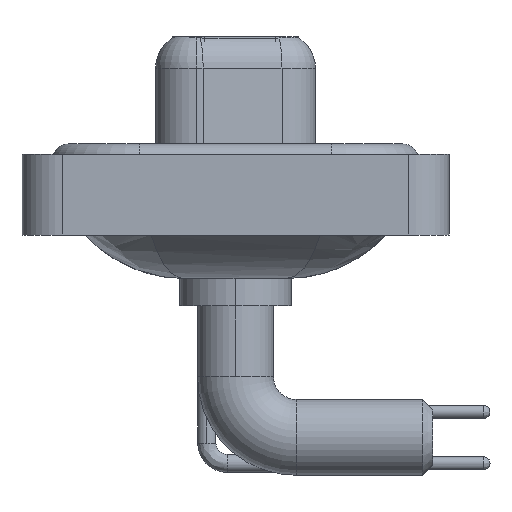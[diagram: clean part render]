
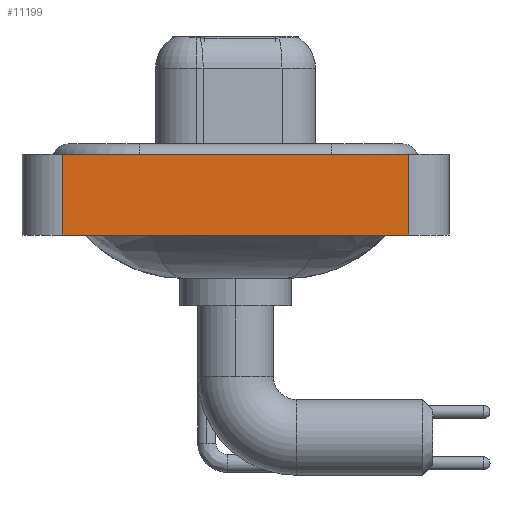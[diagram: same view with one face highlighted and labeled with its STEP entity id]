
A CAD part, left-side view. The second image highlights one B-rep face of the part: STEP entity #11199.
In plain terms, the highlighted planar face has unit normal (-1, 0, 0).
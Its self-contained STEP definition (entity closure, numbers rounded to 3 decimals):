
#631 = VECTOR ( 'NONE', #13515, 1000. ) ;
#1649 = LINE ( 'NONE', #22675, #10372 ) ;
#2010 = DIRECTION ( 'NONE',  ( 0., -1., 0. ) ) ;
#2156 = CARTESIAN_POINT ( 'NONE',  ( -7.35, 8.55, 0.4 ) ) ;
#2305 = VERTEX_POINT ( 'NONE', #13237 ) ;
#2720 = DIRECTION ( 'NONE',  ( 0., 0., 1. ) ) ;
#3395 = EDGE_LOOP ( 'NONE', ( #18081, #11833, #18886, #6422 ) ) ;
#3696 = DIRECTION ( 'NONE',  ( 0., 0., 1. ) ) ;
#4889 = DIRECTION ( 'NONE',  ( 0., -1., 0. ) ) ;
#5348 = LINE ( 'NONE', #7162, #11766 ) ;
#5562 = EDGE_CURVE ( 'NONE', #19245, #2305, #22698, .T. ) ;
#5901 = CARTESIAN_POINT ( 'NONE',  ( -7.35, 8.55, -3.6 ) ) ;
#6056 = CARTESIAN_POINT ( 'NONE',  ( -7.35, -8.55, -3.6 ) ) ;
#6422 = ORIENTED_EDGE ( 'NONE', *, *, #20393, .T. ) ;
#6486 = CARTESIAN_POINT ( 'NONE',  ( -7.35, -8.55, -3.6 ) ) ;
#6576 = CARTESIAN_POINT ( 'NONE',  ( -7.35, -8.55, -3.6 ) ) ;
#6828 = VERTEX_POINT ( 'NONE', #2156 ) ;
#7162 = CARTESIAN_POINT ( 'NONE',  ( -7.35, -8.55, 0.4 ) ) ;
#9732 = CARTESIAN_POINT ( 'NONE',  ( -7.35, -8.55, -3.6 ) ) ;
#10372 = VECTOR ( 'NONE', #3696, 1000. ) ;
#11199 = ADVANCED_FACE ( 'NONE', ( #14770 ), #16617, .T. ) ;
#11508 = VERTEX_POINT ( 'NONE', #5901 ) ;
#11766 = VECTOR ( 'NONE', #2010, 1000. ) ;
#11833 = ORIENTED_EDGE ( 'NONE', *, *, #16425, .F. ) ;
#13062 = DIRECTION ( 'NONE',  ( -1., 0., 0. ) ) ;
#13237 = CARTESIAN_POINT ( 'NONE',  ( -7.35, -8.55, 0.4 ) ) ;
#13515 = DIRECTION ( 'NONE',  ( 0., 0., 1. ) ) ;
#14004 = VECTOR ( 'NONE', #4889, 1000. ) ;
#14770 = FACE_OUTER_BOUND ( 'NONE', #3395, .T. ) ;
#16130 = AXIS2_PLACEMENT_3D ( 'NONE', #6056, #13062, #2720 ) ;
#16425 = EDGE_CURVE ( 'NONE', #6828, #2305, #5348, .T. ) ;
#16617 = PLANE ( 'NONE',  #16130 ) ;
#16948 = LINE ( 'NONE', #9732, #14004 ) ;
#18081 = ORIENTED_EDGE ( 'NONE', *, *, #5562, .T. ) ;
#18108 = EDGE_CURVE ( 'NONE', #11508, #6828, #1649, .T. ) ;
#18886 = ORIENTED_EDGE ( 'NONE', *, *, #18108, .F. ) ;
#19245 = VERTEX_POINT ( 'NONE', #6576 ) ;
#20393 = EDGE_CURVE ( 'NONE', #11508, #19245, #16948, .T. ) ;
#22675 = CARTESIAN_POINT ( 'NONE',  ( -7.35, 8.55, -3.6 ) ) ;
#22698 = LINE ( 'NONE', #6486, #631 ) ;
